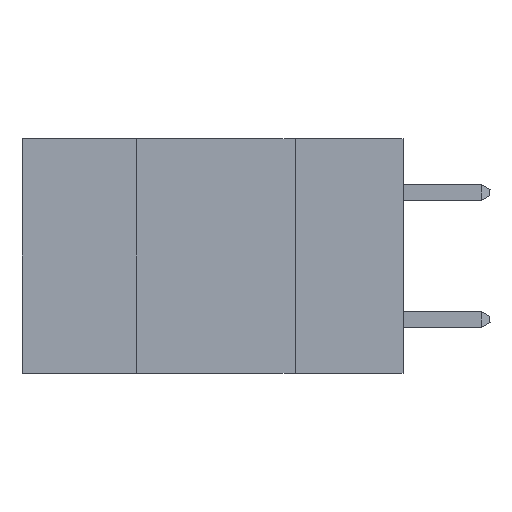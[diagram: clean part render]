
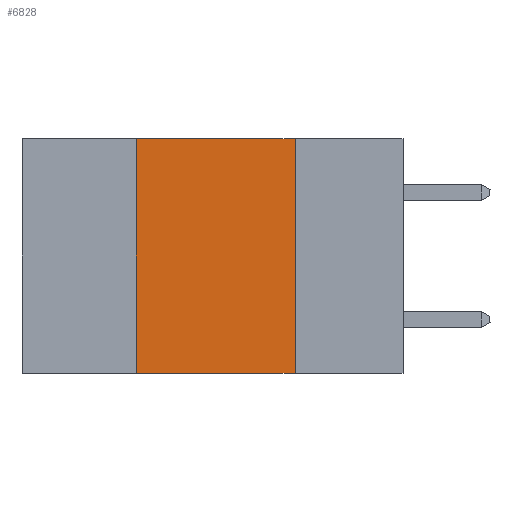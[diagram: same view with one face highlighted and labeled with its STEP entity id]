
A CAD part, left-side view. The second image highlights one B-rep face of the part: STEP entity #6828.
In plain terms, the highlighted planar face has unit normal (-1, 0, 0).
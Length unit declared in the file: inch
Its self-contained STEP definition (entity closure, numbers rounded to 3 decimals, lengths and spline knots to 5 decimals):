
#62 = DIRECTION ( 'NONE',  ( 0., -1., 0. ) ) ;
#554 = VECTOR ( 'NONE', #9297, 39.37008 ) ;
#623 = CARTESIAN_POINT ( 'NONE',  ( 0., 0.6, 0. ) ) ;
#2403 = VERTEX_POINT ( 'NONE', #7859 ) ;
#2669 = DIRECTION ( 'NONE',  ( 0., 0., 1. ) ) ;
#2912 = CARTESIAN_POINT ( 'NONE',  ( 0., 0.42, 0. ) ) ;
#3260 = EDGE_CURVE ( 'NONE', #2403, #11067, #10257, .T. ) ;
#3475 = VECTOR ( 'NONE', #62, 39.37008 ) ;
#3693 = LINE ( 'NONE', #9637, #8178 ) ;
#3785 = EDGE_CURVE ( 'NONE', #8482, #2403, #8210, .T. ) ;
#3788 = LINE ( 'NONE', #4865, #3475 ) ;
#4387 = DIRECTION ( 'NONE',  ( 0., 0., -1. ) ) ;
#4577 = ORIENTED_EDGE ( 'NONE', *, *, #4926, .F. ) ;
#4865 = CARTESIAN_POINT ( 'NONE',  ( 0., 0.6, -0.37 ) ) ;
#4926 = EDGE_CURVE ( 'NONE', #11067, #7182, #3693, .T. ) ;
#5384 = CARTESIAN_POINT ( 'NONE',  ( 0., 0.17, 0. ) ) ;
#5951 = CARTESIAN_POINT ( 'NONE',  ( 0., 0.42, -0.37 ) ) ;
#6159 = CARTESIAN_POINT ( 'NONE',  ( 0., 0.6, 0. ) ) ;
#6601 = DIRECTION ( 'NONE',  ( 0., 0., -1. ) ) ;
#6662 = PLANE ( 'NONE',  #9977 ) ;
#6710 = DIRECTION ( 'NONE',  ( 1., 0., 0. ) ) ;
#6828 = ADVANCED_FACE ( 'NONE', ( #7434 ), #6662, .F. ) ;
#6912 = ORIENTED_EDGE ( 'NONE', *, *, #3260, .F. ) ;
#7182 = VERTEX_POINT ( 'NONE', #8681 ) ;
#7434 = FACE_OUTER_BOUND ( 'NONE', #8092, .T. ) ;
#7859 = CARTESIAN_POINT ( 'NONE',  ( 0., 0.42, 0. ) ) ;
#7915 = VECTOR ( 'NONE', #2669, 39.37008 ) ;
#8092 = EDGE_LOOP ( 'NONE', ( #4577, #6912, #9315, #11467 ) ) ;
#8178 = VECTOR ( 'NONE', #4387, 39.37008 ) ;
#8210 = LINE ( 'NONE', #2912, #7915 ) ;
#8482 = VERTEX_POINT ( 'NONE', #5951 ) ;
#8681 = CARTESIAN_POINT ( 'NONE',  ( 0., 0.17, -0.37 ) ) ;
#9147 = EDGE_CURVE ( 'NONE', #8482, #7182, #3788, .T. ) ;
#9297 = DIRECTION ( 'NONE',  ( 0., -1., 0. ) ) ;
#9315 = ORIENTED_EDGE ( 'NONE', *, *, #3785, .F. ) ;
#9637 = CARTESIAN_POINT ( 'NONE',  ( 0., 0.17, 0. ) ) ;
#9977 = AXIS2_PLACEMENT_3D ( 'NONE', #6159, #6710, #6601 ) ;
#10257 = LINE ( 'NONE', #623, #554 ) ;
#11067 = VERTEX_POINT ( 'NONE', #5384 ) ;
#11467 = ORIENTED_EDGE ( 'NONE', *, *, #9147, .T. ) ;
